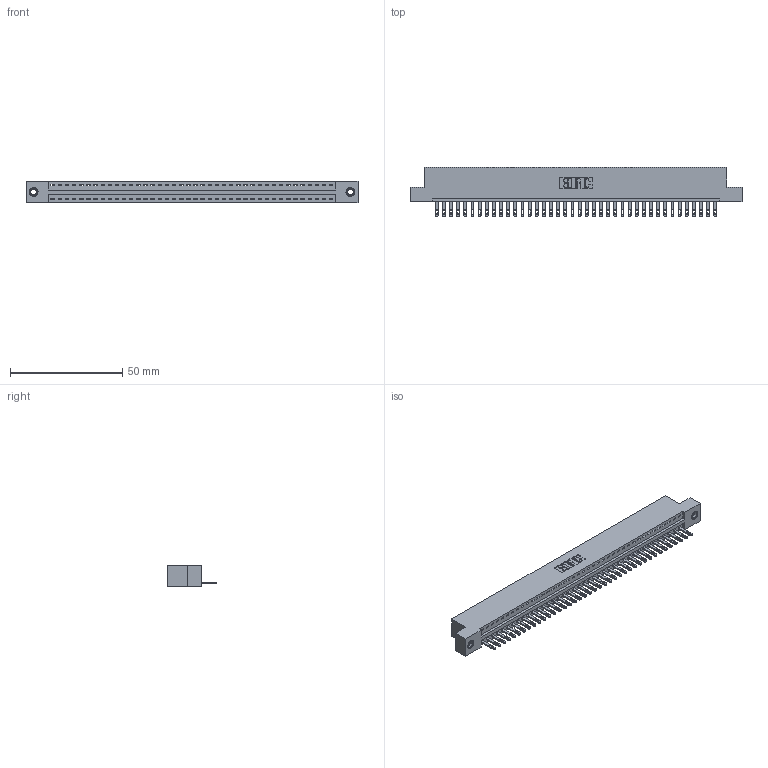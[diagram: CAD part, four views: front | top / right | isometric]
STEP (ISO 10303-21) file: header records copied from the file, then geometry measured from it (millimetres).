
FILE_DESCRIPTION (( 'STEP AP203' ), '1' );
FILE_NAME ('346-040-500-107.STEP', '2022-05-07T08:23:43', ( '' ), ( '' ), 'SwSTEP 2.0', 'SolidWorks 2020', '' );
FILE_SCHEMA (( 'CONFIG_CONTROL_DESIGN' ));
Length unit declared in the file: inch
Products named in the file (4): 345-292-001_345-293-100; 345-250-001_345-250-005-103; 346 Part_Flush Mounting Lugs - 0.156 Dia-TI; 346-040-500-107
Assembly tree (43 placements, depth 2):
  346-040-500-107
    346 Part_Flush Mounting Lugs - 0.156 Dia-TI
    345-292-001_345-293-100  x40
    345-250-001_345-250-005-103  x2
Bounding box: 147.57 x 21.84 x 9.4 mm (x, y, z)
Volume: 14123.6 mm3; surface area: 17758.9 mm2
Topology: 43 solids, 43 shells, 2342 faces, 7185 edges, 4782 vertices
Faces by surface type: plane 1468, cylinder 858, cone 12, torus 4
Entity records: 26210 total; most frequent: CARTESIAN_POINT 4475, ORIENTED_EDGE 4442, DIRECTION 3979, EDGE_CURVE 2221, VECTOR 1905, LINE 1905, VERTEX_POINT 1476, AXIS2_PLACEMENT_3D 1037
